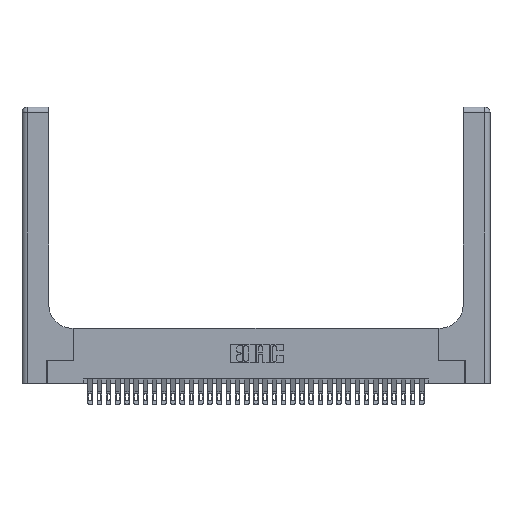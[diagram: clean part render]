
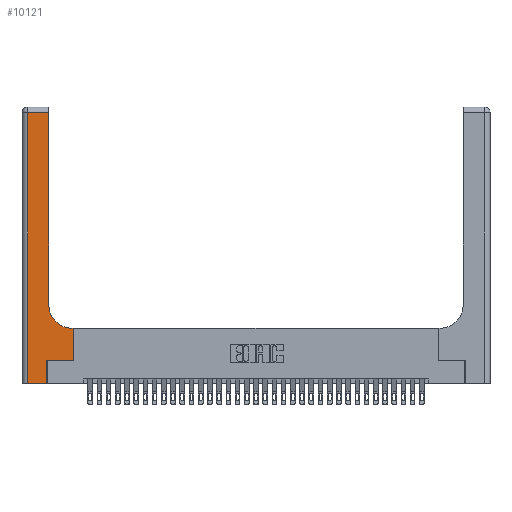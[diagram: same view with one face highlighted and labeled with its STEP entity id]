
A CAD part, top view. The second image highlights one B-rep face of the part: STEP entity #10121.
In plain terms, the highlighted planar face has unit normal (0, 0, 1).
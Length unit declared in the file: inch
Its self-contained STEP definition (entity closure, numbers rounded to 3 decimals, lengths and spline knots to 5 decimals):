
#143 = VERTEX_POINT ( 'NONE', #18720 ) ;
#362 = CARTESIAN_POINT ( 'NONE',  ( 0., 2.94, 0.37 ) ) ;
#692 = VECTOR ( 'NONE', #15031, 39.37008 ) ;
#811 = ORIENTED_EDGE ( 'NONE', *, *, #14191, .T. ) ;
#1906 = LINE ( 'NONE', #362, #18415 ) ;
#4251 = DIRECTION ( 'NONE',  ( 1., 0., 0. ) ) ;
#4970 = CARTESIAN_POINT ( 'NONE',  ( 0., 3., 0.37 ) ) ;
#5421 = ORIENTED_EDGE ( 'NONE', *, *, #25049, .T. ) ;
#6560 = DIRECTION ( 'NONE',  ( 0., 1., 0. ) ) ;
#6954 = EDGE_CURVE ( 'NONE', #32910, #10726, #29063, .T. ) ;
#7403 = CARTESIAN_POINT ( 'NONE',  ( 0.06, 2.94, 0.37 ) ) ;
#7915 = CARTESIAN_POINT ( 'NONE',  ( 0.269, 0., 0.37 ) ) ;
#7945 = ORIENTED_EDGE ( 'NONE', *, *, #30840, .T. ) ;
#8789 = LINE ( 'NONE', #33549, #31840 ) ;
#9506 = CARTESIAN_POINT ( 'NONE',  ( 0.2915, 0.85, 0.37 ) ) ;
#10047 = CARTESIAN_POINT ( 'NONE',  ( 0.2915, 0.6, 0.37 ) ) ;
#10121 = ADVANCED_FACE ( 'NONE', ( #27473 ), #14445, .F. ) ;
#10258 = VECTOR ( 'NONE', #4251, 39.37008 ) ;
#10613 = CARTESIAN_POINT ( 'NONE',  ( 0.5585, 0.25, 0.37 ) ) ;
#10726 = VERTEX_POINT ( 'NONE', #9506 ) ;
#10823 = CARTESIAN_POINT ( 'NONE',  ( 0.5415, 0.6, 0.37 ) ) ;
#10834 = EDGE_CURVE ( 'NONE', #17107, #16041, #24046, .T. ) ;
#10910 = ORIENTED_EDGE ( 'NONE', *, *, #23420, .T. ) ;
#11180 = ORIENTED_EDGE ( 'NONE', *, *, #17087, .T. ) ;
#11683 = CARTESIAN_POINT ( 'NONE',  ( 0.5585, 0.6, 0.37 ) ) ;
#12276 = ORIENTED_EDGE ( 'NONE', *, *, #25417, .T. ) ;
#12835 = LINE ( 'NONE', #19159, #16604 ) ;
#12872 = VERTEX_POINT ( 'NONE', #7915 ) ;
#13458 = DIRECTION ( 'NONE',  ( 0., 1., 0. ) ) ;
#13463 = CARTESIAN_POINT ( 'NONE',  ( 0.06, 0., 0.37 ) ) ;
#14191 = EDGE_CURVE ( 'NONE', #32299, #12872, #34506, .T. ) ;
#14445 = PLANE ( 'NONE',  #34277 ) ;
#15012 = DIRECTION ( 'NONE',  ( -1., 0., 0. ) ) ;
#15031 = DIRECTION ( 'NONE',  ( 1., 0., 0. ) ) ;
#15762 = ORIENTED_EDGE ( 'NONE', *, *, #6954, .T. ) ;
#15763 = DIRECTION ( 'NONE',  ( 0., 0., -1. ) ) ;
#16041 = VERTEX_POINT ( 'NONE', #11683 ) ;
#16566 = EDGE_CURVE ( 'NONE', #21098, #17107, #24162, .T. ) ;
#16604 = VECTOR ( 'NONE', #6560, 39.37008 ) ;
#16764 = ORIENTED_EDGE ( 'NONE', *, *, #16566, .T. ) ;
#17087 = EDGE_CURVE ( 'NONE', #32861, #32299, #8789, .T. ) ;
#17107 = VERTEX_POINT ( 'NONE', #10613 ) ;
#17204 = DIRECTION ( 'NONE',  ( 0., -1., 0. ) ) ;
#17461 = ORIENTED_EDGE ( 'NONE', *, *, #10834, .T. ) ;
#18346 = LINE ( 'NONE', #10047, #22171 ) ;
#18415 = VECTOR ( 'NONE', #19399, 39.37008 ) ;
#18720 = CARTESIAN_POINT ( 'NONE',  ( 0.2915, 2.94, 0.37 ) ) ;
#18838 = CARTESIAN_POINT ( 'NONE',  ( 0.2915, 3., 0.37 ) ) ;
#19159 = CARTESIAN_POINT ( 'NONE',  ( 0.269, 0., 0.37 ) ) ;
#19399 = DIRECTION ( 'NONE',  ( -1., 0., 0. ) ) ;
#21098 = VERTEX_POINT ( 'NONE', #34956 ) ;
#22171 = VECTOR ( 'NONE', #15012, 39.37008 ) ;
#23089 = CARTESIAN_POINT ( 'NONE',  ( 0., 0., 0.37 ) ) ;
#23420 = EDGE_CURVE ( 'NONE', #143, #32861, #1906, .T. ) ;
#24046 = LINE ( 'NONE', #26753, #30438 ) ;
#24162 = LINE ( 'NONE', #30293, #692 ) ;
#24248 = EDGE_LOOP ( 'NONE', ( #12276, #10910, #11180, #811, #5421, #16764, #17461, #7945, #15762 ) ) ;
#25049 = EDGE_CURVE ( 'NONE', #12872, #21098, #12835, .T. ) ;
#25417 = EDGE_CURVE ( 'NONE', #10726, #143, #33230, .T. ) ;
#26752 = CARTESIAN_POINT ( 'NONE',  ( 0.5415, 0.85, 0.37 ) ) ;
#26753 = CARTESIAN_POINT ( 'NONE',  ( 0.5585, 0.25, 0.37 ) ) ;
#26832 = VECTOR ( 'NONE', #32815, 39.37008 ) ;
#26992 = DIRECTION ( 'NONE',  ( 1., 0., 0. ) ) ;
#27473 = FACE_OUTER_BOUND ( 'NONE', #24248, .T. ) ;
#29063 = CIRCLE ( 'NONE', #33069, 0.25 ) ;
#30293 = CARTESIAN_POINT ( 'NONE',  ( 0.269, 0.25, 0.37 ) ) ;
#30438 = VECTOR ( 'NONE', #13458, 39.37008 ) ;
#30840 = EDGE_CURVE ( 'NONE', #16041, #32910, #18346, .T. ) ;
#31840 = VECTOR ( 'NONE', #17204, 39.37008 ) ;
#32179 = DIRECTION ( 'NONE',  ( 0., 0., -1. ) ) ;
#32225 = DIRECTION ( 'NONE',  ( -1., 0., 0. ) ) ;
#32299 = VERTEX_POINT ( 'NONE', #13463 ) ;
#32815 = DIRECTION ( 'NONE',  ( 0., 1., 0. ) ) ;
#32861 = VERTEX_POINT ( 'NONE', #7403 ) ;
#32910 = VERTEX_POINT ( 'NONE', #10823 ) ;
#33069 = AXIS2_PLACEMENT_3D ( 'NONE', #26752, #32179, #26992 ) ;
#33230 = LINE ( 'NONE', #18838, #26832 ) ;
#33549 = CARTESIAN_POINT ( 'NONE',  ( 0.06, 3., 0.37 ) ) ;
#34277 = AXIS2_PLACEMENT_3D ( 'NONE', #4970, #15763, #32225 ) ;
#34506 = LINE ( 'NONE', #23089, #10258 ) ;
#34956 = CARTESIAN_POINT ( 'NONE',  ( 0.269, 0.25, 0.37 ) ) ;
